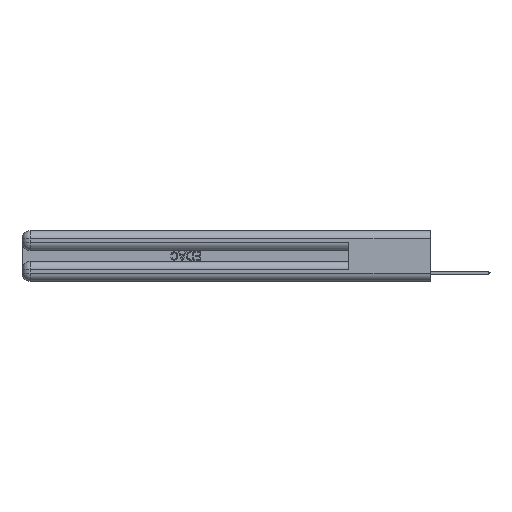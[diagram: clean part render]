
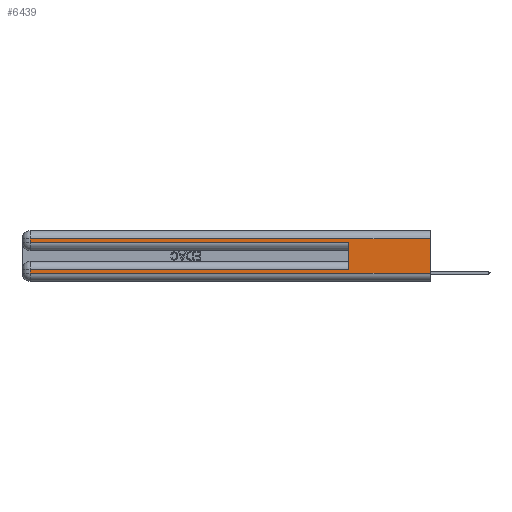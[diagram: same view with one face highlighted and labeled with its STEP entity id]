
A CAD part, left-side view. The second image highlights one B-rep face of the part: STEP entity #6439.
In plain terms, the highlighted planar face has unit normal (-1, 0, 0).
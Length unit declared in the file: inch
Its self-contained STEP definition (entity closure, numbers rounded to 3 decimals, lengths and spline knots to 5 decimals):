
#718 = VERTEX_POINT ( 'NONE', #20630 ) ;
#1556 = FACE_OUTER_BOUND ( 'NONE', #12214, .T. ) ;
#2082 = ORIENTED_EDGE ( 'NONE', *, *, #31925, .T. ) ;
#2748 = CARTESIAN_POINT ( 'NONE',  ( 0., 0.6, 0.085 ) ) ;
#2766 = ORIENTED_EDGE ( 'NONE', *, *, #18857, .T. ) ;
#2837 = DIRECTION ( 'NONE',  ( 0., -1., 0. ) ) ;
#4173 = ORIENTED_EDGE ( 'NONE', *, *, #30497, .T. ) ;
#4503 = LINE ( 'NONE', #25885, #14752 ) ;
#4522 = ORIENTED_EDGE ( 'NONE', *, *, #25149, .F. ) ;
#4562 = DIRECTION ( 'NONE',  ( 0., -1., 0. ) ) ;
#4614 = VECTOR ( 'NONE', #4562, 39.37008 ) ;
#4682 = VECTOR ( 'NONE', #20609, 39.37008 ) ;
#5428 = LINE ( 'NONE', #26458, #15796 ) ;
#5797 = LINE ( 'NONE', #32528, #30971 ) ;
#6105 = CARTESIAN_POINT ( 'NONE',  ( 0., 0., 0.06 ) ) ;
#6439 = ADVANCED_FACE ( 'NONE', ( #1556 ), #7081, .F. ) ;
#7081 = PLANE ( 'NONE',  #25460 ) ;
#7183 = EDGE_CURVE ( 'NONE', #16770, #26479, #28482, .T. ) ;
#7801 = ORIENTED_EDGE ( 'NONE', *, *, #16844, .T. ) ;
#7928 = DIRECTION ( 'NONE',  ( 0., 0., -1. ) ) ;
#8872 = VERTEX_POINT ( 'NONE', #2748 ) ;
#9459 = ORIENTED_EDGE ( 'NONE', *, *, #23332, .T. ) ;
#9574 = CARTESIAN_POINT ( 'NONE',  ( 0., 2.94, 0.085 ) ) ;
#10078 = LINE ( 'NONE', #20434, #4682 ) ;
#12214 = EDGE_LOOP ( 'NONE', ( #26860, #28731, #9459, #7801, #4522, #4173, #2766, #2082 ) ) ;
#12894 = LINE ( 'NONE', #20666, #13802 ) ;
#13743 = VERTEX_POINT ( 'NONE', #24474 ) ;
#13802 = VECTOR ( 'NONE', #16014, 39.37008 ) ;
#14752 = VECTOR ( 'NONE', #17968, 39.37008 ) ;
#15193 = DIRECTION ( 'NONE',  ( 0., 0., -1. ) ) ;
#15635 = VECTOR ( 'NONE', #15193, 39.37008 ) ;
#15740 = EDGE_CURVE ( 'NONE', #16770, #27075, #4503, .T. ) ;
#15796 = VECTOR ( 'NONE', #2837, 39.37008 ) ;
#16014 = DIRECTION ( 'NONE',  ( 0., 0., -1. ) ) ;
#16770 = VERTEX_POINT ( 'NONE', #26982 ) ;
#16844 = EDGE_CURVE ( 'NONE', #13743, #24363, #5428, .T. ) ;
#16956 = LINE ( 'NONE', #23454, #21942 ) ;
#17599 = DIRECTION ( 'NONE',  ( 1., 0., 0. ) ) ;
#17968 = DIRECTION ( 'NONE',  ( 0., 1., 0. ) ) ;
#18857 = EDGE_CURVE ( 'NONE', #30436, #718, #16956, .T. ) ;
#20434 = CARTESIAN_POINT ( 'NONE',  ( 0., 0., 0.085 ) ) ;
#20609 = DIRECTION ( 'NONE',  ( 0., 1., 0. ) ) ;
#20630 = CARTESIAN_POINT ( 'NONE',  ( 0., 2.94, 0.06 ) ) ;
#20666 = CARTESIAN_POINT ( 'NONE',  ( 0., 2.94, 0.37 ) ) ;
#21942 = VECTOR ( 'NONE', #7928, 39.37008 ) ;
#22350 = LINE ( 'NONE', #33047, #4614 ) ;
#23332 = EDGE_CURVE ( 'NONE', #27075, #13743, #12894, .T. ) ;
#23454 = CARTESIAN_POINT ( 'NONE',  ( 0., 2.94, 0.37 ) ) ;
#24363 = VERTEX_POINT ( 'NONE', #27426 ) ;
#24474 = CARTESIAN_POINT ( 'NONE',  ( 0., 2.94, 0.285 ) ) ;
#24750 = DIRECTION ( 'NONE',  ( 0., 0., 1. ) ) ;
#25149 = EDGE_CURVE ( 'NONE', #8872, #24363, #5797, .T. ) ;
#25460 = AXIS2_PLACEMENT_3D ( 'NONE', #27949, #17599, #31229 ) ;
#25885 = CARTESIAN_POINT ( 'NONE',  ( 0., 0., 0.31 ) ) ;
#26458 = CARTESIAN_POINT ( 'NONE',  ( 0., 0., 0.285 ) ) ;
#26479 = VERTEX_POINT ( 'NONE', #6105 ) ;
#26860 = ORIENTED_EDGE ( 'NONE', *, *, #7183, .F. ) ;
#26982 = CARTESIAN_POINT ( 'NONE',  ( 0., 0., 0.31 ) ) ;
#27075 = VERTEX_POINT ( 'NONE', #32909 ) ;
#27426 = CARTESIAN_POINT ( 'NONE',  ( 0., 0.6, 0.285 ) ) ;
#27949 = CARTESIAN_POINT ( 'NONE',  ( 0., 0., 0.37 ) ) ;
#28482 = LINE ( 'NONE', #31073, #15635 ) ;
#28731 = ORIENTED_EDGE ( 'NONE', *, *, #15740, .T. ) ;
#30436 = VERTEX_POINT ( 'NONE', #9574 ) ;
#30497 = EDGE_CURVE ( 'NONE', #8872, #30436, #10078, .T. ) ;
#30971 = VECTOR ( 'NONE', #24750, 39.37008 ) ;
#31073 = CARTESIAN_POINT ( 'NONE',  ( 0., 0., 0.37 ) ) ;
#31229 = DIRECTION ( 'NONE',  ( 0., 0., -1. ) ) ;
#31925 = EDGE_CURVE ( 'NONE', #718, #26479, #22350, .T. ) ;
#32528 = CARTESIAN_POINT ( 'NONE',  ( 0., 0.6, 0.145 ) ) ;
#32909 = CARTESIAN_POINT ( 'NONE',  ( 0., 2.94, 0.31 ) ) ;
#33047 = CARTESIAN_POINT ( 'NONE',  ( 0., 0., 0.06 ) ) ;
